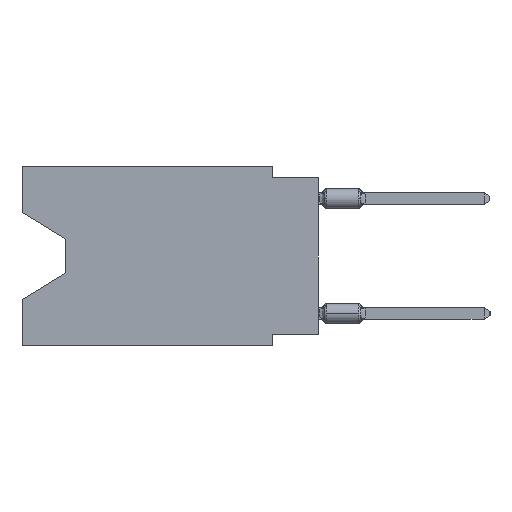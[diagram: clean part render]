
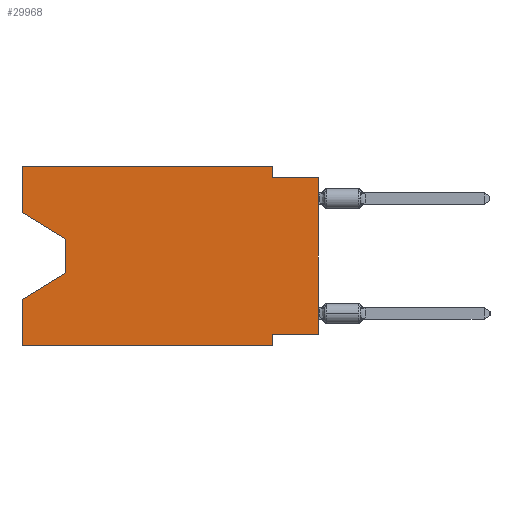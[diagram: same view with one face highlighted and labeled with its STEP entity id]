
A CAD part, left-side view. The second image highlights one B-rep face of the part: STEP entity #29968.
In plain terms, the highlighted planar face has unit normal (-1, 0, 0).
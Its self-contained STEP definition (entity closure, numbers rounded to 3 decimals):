
#92 = CARTESIAN_POINT ( 'NONE',  ( 0., 16.383, -9.906 ) ) ;
#123 = CARTESIAN_POINT ( 'NONE',  ( 0., 16.383, 0. ) ) ;
#199 = EDGE_CURVE ( 'NONE', #8684, #17775, #35908, .T. ) ;
#230 = LINE ( 'NONE', #10403, #22013 ) ;
#382 = ORIENTED_EDGE ( 'NONE', *, *, #3711, .F. ) ;
#555 = DIRECTION ( 'NONE',  ( 0., -0.855, -0.519 ) ) ;
#1611 = LINE ( 'NONE', #4487, #22575 ) ;
#1660 = LINE ( 'NONE', #38482, #17205 ) ;
#1753 = CARTESIAN_POINT ( 'NONE',  ( 0., 16.383, -9.906 ) ) ;
#2117 = VERTEX_POINT ( 'NONE', #30942 ) ;
#3291 = ORIENTED_EDGE ( 'NONE', *, *, #23666, .F. ) ;
#3711 = EDGE_CURVE ( 'NONE', #30872, #41140, #16633, .T. ) ;
#3849 = ORIENTED_EDGE ( 'NONE', *, *, #19083, .T. ) ;
#4005 = CARTESIAN_POINT ( 'NONE',  ( 0., 16.383, 0. ) ) ;
#4451 = VECTOR ( 'NONE', #8272, 1000. ) ;
#4487 = CARTESIAN_POINT ( 'NONE',  ( 0., 13.97, -4.013 ) ) ;
#4658 = LINE ( 'NONE', #92, #15342 ) ;
#5524 = CARTESIAN_POINT ( 'NONE',  ( 0., 0., 0. ) ) ;
#6038 = EDGE_CURVE ( 'NONE', #2117, #28603, #1660, .T. ) ;
#6051 = VECTOR ( 'NONE', #29115, 1000. ) ;
#6591 = ORIENTED_EDGE ( 'NONE', *, *, #31550, .F. ) ;
#7332 = CARTESIAN_POINT ( 'NONE',  ( 0., 16.383, 0. ) ) ;
#8272 = DIRECTION ( 'NONE',  ( 0., -1., 0. ) ) ;
#8323 = LINE ( 'NONE', #25829, #18255 ) ;
#8684 = VERTEX_POINT ( 'NONE', #36675 ) ;
#8710 = CARTESIAN_POINT ( 'NONE',  ( 0., 0., -9.271 ) ) ;
#9872 = VECTOR ( 'NONE', #40792, 1000. ) ;
#10368 = VERTEX_POINT ( 'NONE', #4005 ) ;
#10403 = CARTESIAN_POINT ( 'NONE',  ( 0., 16.383, 0. ) ) ;
#10904 = ORIENTED_EDGE ( 'NONE', *, *, #43823, .F. ) ;
#12365 = ORIENTED_EDGE ( 'NONE', *, *, #21683, .F. ) ;
#12544 = EDGE_CURVE ( 'NONE', #21971, #38244, #4658, .T. ) ;
#13181 = PLANE ( 'NONE',  #15186 ) ;
#13492 = CARTESIAN_POINT ( 'NONE',  ( 0., 13.97, -4.013 ) ) ;
#13798 = VECTOR ( 'NONE', #23089, 1000. ) ;
#14409 = DIRECTION ( 'NONE',  ( 0., 0., 1. ) ) ;
#14846 = EDGE_CURVE ( 'NONE', #35692, #38244, #8323, .T. ) ;
#15137 = LINE ( 'NONE', #8710, #6051 ) ;
#15171 = DIRECTION ( 'NONE',  ( 0., 0.855, -0.519 ) ) ;
#15186 = AXIS2_PLACEMENT_3D ( 'NONE', #123, #37587, #30919 ) ;
#15342 = VECTOR ( 'NONE', #38370, 1000. ) ;
#16633 = LINE ( 'NONE', #30388, #13798 ) ;
#17087 = ORIENTED_EDGE ( 'NONE', *, *, #36686, .F. ) ;
#17205 = VECTOR ( 'NONE', #15171, 1000. ) ;
#17274 = CARTESIAN_POINT ( 'NONE',  ( 0., 2.54, -9.906 ) ) ;
#17775 = VERTEX_POINT ( 'NONE', #31766 ) ;
#18255 = VECTOR ( 'NONE', #28501, 1000. ) ;
#19083 = EDGE_CURVE ( 'NONE', #35321, #2117, #1611, .T. ) ;
#19844 = CARTESIAN_POINT ( 'NONE',  ( 0., 16.383, -2.546 ) ) ;
#21260 = LINE ( 'NONE', #27265, #9872 ) ;
#21683 = EDGE_CURVE ( 'NONE', #10368, #30872, #230, .T. ) ;
#21971 = VERTEX_POINT ( 'NONE', #1753 ) ;
#22013 = VECTOR ( 'NONE', #23959, 1000. ) ;
#22213 = EDGE_LOOP ( 'NONE', ( #23328, #3849, #37431, #3291, #33474, #38769, #6591, #25754, #10904, #382, #12365, #17087 ) ) ;
#22575 = VECTOR ( 'NONE', #28663, 1000. ) ;
#23089 = DIRECTION ( 'NONE',  ( 0., 0., -1. ) ) ;
#23328 = ORIENTED_EDGE ( 'NONE', *, *, #40381, .T. ) ;
#23666 = EDGE_CURVE ( 'NONE', #21971, #28603, #21260, .T. ) ;
#23959 = DIRECTION ( 'NONE',  ( 0., -1., 0. ) ) ;
#25031 = CARTESIAN_POINT ( 'NONE',  ( 0., 2.54, 0. ) ) ;
#25627 = CARTESIAN_POINT ( 'NONE',  ( 0., 16.383, -7.36 ) ) ;
#25754 = ORIENTED_EDGE ( 'NONE', *, *, #199, .T. ) ;
#25778 = CARTESIAN_POINT ( 'NONE',  ( 0., 0., -0.635 ) ) ;
#25829 = CARTESIAN_POINT ( 'NONE',  ( 0., 2.54, -9.906 ) ) ;
#26191 = VECTOR ( 'NONE', #14409, 1000. ) ;
#27265 = CARTESIAN_POINT ( 'NONE',  ( 0., 16.383, 0. ) ) ;
#28183 = LINE ( 'NONE', #7332, #26191 ) ;
#28428 = VECTOR ( 'NONE', #555, 1000. ) ;
#28501 = DIRECTION ( 'NONE',  ( 0., 0., -1. ) ) ;
#28603 = VERTEX_POINT ( 'NONE', #25627 ) ;
#28663 = DIRECTION ( 'NONE',  ( 0., 0., -1. ) ) ;
#29115 = DIRECTION ( 'NONE',  ( 0., 1., 0. ) ) ;
#29218 = CARTESIAN_POINT ( 'NONE',  ( 0., 2.54, -0.635 ) ) ;
#29427 = CARTESIAN_POINT ( 'NONE',  ( 0., 2.54, -9.271 ) ) ;
#29968 = ADVANCED_FACE ( 'NONE', ( #33823 ), #13181, .F. ) ;
#30388 = CARTESIAN_POINT ( 'NONE',  ( 0., 2.54, 0. ) ) ;
#30700 = LINE ( 'NONE', #19844, #28428 ) ;
#30872 = VERTEX_POINT ( 'NONE', #25031 ) ;
#30919 = DIRECTION ( 'NONE',  ( 0., 0., -1. ) ) ;
#30942 = CARTESIAN_POINT ( 'NONE',  ( 0., 13.97, -5.893 ) ) ;
#31550 = EDGE_CURVE ( 'NONE', #8684, #35692, #15137, .T. ) ;
#31766 = CARTESIAN_POINT ( 'NONE',  ( 0., 0., -0.635 ) ) ;
#33474 = ORIENTED_EDGE ( 'NONE', *, *, #12544, .T. ) ;
#33823 = FACE_OUTER_BOUND ( 'NONE', #22213, .T. ) ;
#35321 = VERTEX_POINT ( 'NONE', #13492 ) ;
#35692 = VERTEX_POINT ( 'NONE', #29427 ) ;
#35908 = LINE ( 'NONE', #5524, #36151 ) ;
#36151 = VECTOR ( 'NONE', #42111, 1000. ) ;
#36210 = LINE ( 'NONE', #25778, #4451 ) ;
#36675 = CARTESIAN_POINT ( 'NONE',  ( 0., 0., -9.271 ) ) ;
#36686 = EDGE_CURVE ( 'NONE', #41437, #10368, #28183, .T. ) ;
#37431 = ORIENTED_EDGE ( 'NONE', *, *, #6038, .T. ) ;
#37587 = DIRECTION ( 'NONE',  ( 1., 0., 0. ) ) ;
#38244 = VERTEX_POINT ( 'NONE', #17274 ) ;
#38298 = CARTESIAN_POINT ( 'NONE',  ( 0., 16.383, -2.546 ) ) ;
#38370 = DIRECTION ( 'NONE',  ( 0., -1., 0. ) ) ;
#38482 = CARTESIAN_POINT ( 'NONE',  ( 0., 13.97, -5.893 ) ) ;
#38769 = ORIENTED_EDGE ( 'NONE', *, *, #14846, .F. ) ;
#40381 = EDGE_CURVE ( 'NONE', #41437, #35321, #30700, .T. ) ;
#40792 = DIRECTION ( 'NONE',  ( 0., 0., 1. ) ) ;
#41140 = VERTEX_POINT ( 'NONE', #29218 ) ;
#41437 = VERTEX_POINT ( 'NONE', #38298 ) ;
#42111 = DIRECTION ( 'NONE',  ( 0., 0., 1. ) ) ;
#43823 = EDGE_CURVE ( 'NONE', #41140, #17775, #36210, .T. ) ;
